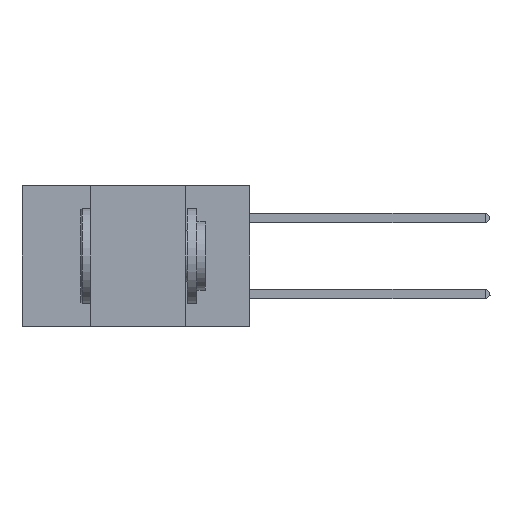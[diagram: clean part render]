
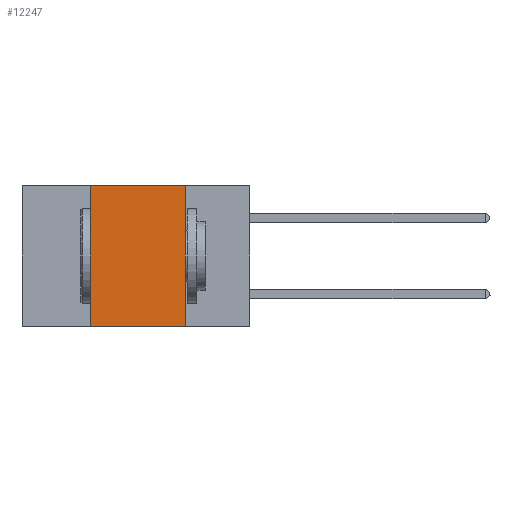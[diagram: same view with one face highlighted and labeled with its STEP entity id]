
A CAD part, left-side view. The second image highlights one B-rep face of the part: STEP entity #12247.
In plain terms, the highlighted planar face has unit normal (-1, 0, 0).
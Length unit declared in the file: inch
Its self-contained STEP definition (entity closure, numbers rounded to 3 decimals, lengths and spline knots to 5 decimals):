
#83 = DIRECTION ( 'NONE',  ( 0., 0., -1. ) ) ;
#139 = AXIS2_PLACEMENT_3D ( 'NONE', #6893, #8411, #18704 ) ;
#168 = ORIENTED_EDGE ( 'NONE', *, *, #5988, .F. ) ;
#846 = CARTESIAN_POINT ( 'NONE',  ( 0., 0.17, 0. ) ) ;
#2034 = CARTESIAN_POINT ( 'NONE',  ( 0., 0.42, 0. ) ) ;
#2433 = VERTEX_POINT ( 'NONE', #7750 ) ;
#2710 = EDGE_LOOP ( 'NONE', ( #2919, #3880, #168, #12339 ) ) ;
#2919 = ORIENTED_EDGE ( 'NONE', *, *, #15350, .F. ) ;
#3264 = CARTESIAN_POINT ( 'NONE',  ( 0., 0.17, -0.37 ) ) ;
#3849 = EDGE_CURVE ( 'NONE', #2433, #9025, #13044, .T. ) ;
#3880 = ORIENTED_EDGE ( 'NONE', *, *, #16058, .F. ) ;
#4855 = DIRECTION ( 'NONE',  ( 0., -1., 0. ) ) ;
#4856 = DIRECTION ( 'NONE',  ( 0., -1., 0. ) ) ;
#5138 = CARTESIAN_POINT ( 'NONE',  ( 0., 0.6, -0.37 ) ) ;
#5697 = DIRECTION ( 'NONE',  ( 0., 0., 1. ) ) ;
#5988 = EDGE_CURVE ( 'NONE', #2433, #18782, #12723, .T. ) ;
#6893 = CARTESIAN_POINT ( 'NONE',  ( 0., 0.6, 0. ) ) ;
#7750 = CARTESIAN_POINT ( 'NONE',  ( 0., 0.42, -0.37 ) ) ;
#8411 = DIRECTION ( 'NONE',  ( 1., 0., 0. ) ) ;
#9025 = VERTEX_POINT ( 'NONE', #3264 ) ;
#9109 = VECTOR ( 'NONE', #4856, 39.37008 ) ;
#9985 = FACE_OUTER_BOUND ( 'NONE', #2710, .T. ) ;
#10278 = CARTESIAN_POINT ( 'NONE',  ( 0., 0.42, 0. ) ) ;
#12247 = ADVANCED_FACE ( 'NONE', ( #9985 ), #15760, .F. ) ;
#12334 = CARTESIAN_POINT ( 'NONE',  ( 0., 0.6, 0. ) ) ;
#12339 = ORIENTED_EDGE ( 'NONE', *, *, #3849, .T. ) ;
#12723 = LINE ( 'NONE', #10278, #15524 ) ;
#13044 = LINE ( 'NONE', #5138, #9109 ) ;
#13688 = VERTEX_POINT ( 'NONE', #846 ) ;
#15350 = EDGE_CURVE ( 'NONE', #13688, #9025, #17171, .T. ) ;
#15524 = VECTOR ( 'NONE', #5697, 39.37008 ) ;
#15555 = VECTOR ( 'NONE', #4855, 39.37008 ) ;
#15760 = PLANE ( 'NONE',  #139 ) ;
#15993 = LINE ( 'NONE', #12334, #15555 ) ;
#16058 = EDGE_CURVE ( 'NONE', #18782, #13688, #15993, .T. ) ;
#16695 = VECTOR ( 'NONE', #83, 39.37008 ) ;
#17171 = LINE ( 'NONE', #18120, #16695 ) ;
#18120 = CARTESIAN_POINT ( 'NONE',  ( 0., 0.17, 0. ) ) ;
#18704 = DIRECTION ( 'NONE',  ( 0., 0., -1. ) ) ;
#18782 = VERTEX_POINT ( 'NONE', #2034 ) ;
